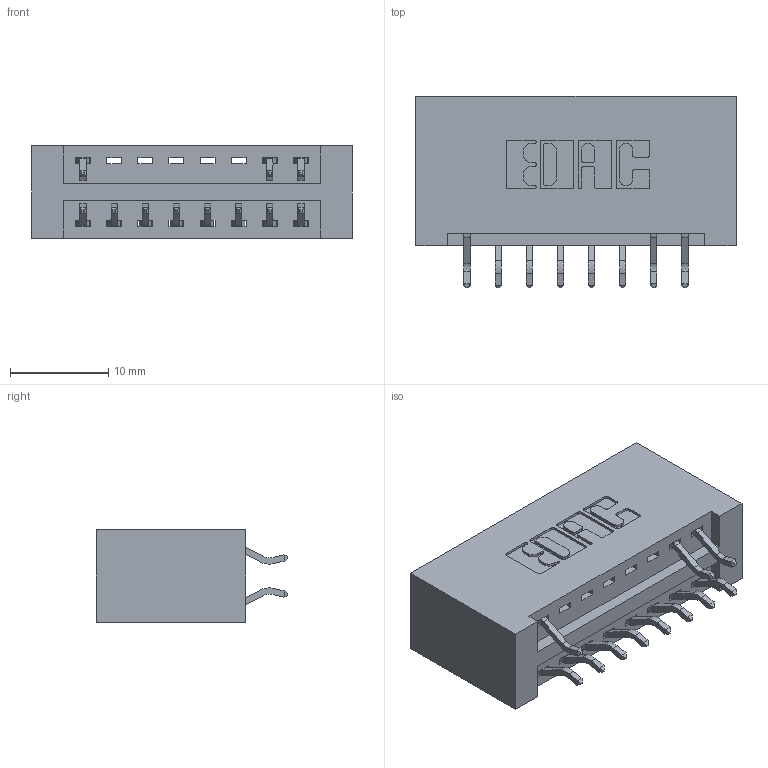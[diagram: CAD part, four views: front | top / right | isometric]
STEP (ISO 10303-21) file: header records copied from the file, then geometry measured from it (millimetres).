
FILE_DESCRIPTION (( 'STEP AP203' ), '1' );
FILE_NAME ('346-016-556-201.STEP', '2018-08-20T04:55:42', ( '' ), ( '' ), 'SwSTEP 2.0', 'SolidWorks 2016', '' );
FILE_SCHEMA (( 'CONFIG_CONTROL_DESIGN' ));
Length unit declared in the file: inch
Products named in the file (3): 346 Part_No Mounting Lugs; 345-292-001_556 Tail; 346-016-556-201
Assembly tree (12 placements, depth 2):
  346-016-556-201
    346 Part_No Mounting Lugs
    345-292-001_556 Tail  x11
Bounding box: 32.64 x 19.57 x 9.4 mm (x, y, z)
Volume: 3446.5 mm3; surface area: 4096.5 mm2
Topology: 12 solids, 12 shells, 782 faces, 2313 edges, 1526 vertices
Faces by surface type: plane 526, cylinder 256
Entity records: 9581 total; most frequent: CARTESIAN_POINT 1659, ORIENTED_EDGE 1586, DIRECTION 1491, EDGE_CURVE 793, VECTOR 629, LINE 629, VERTEX_POINT 526, AXIS2_PLACEMENT_3D 431
